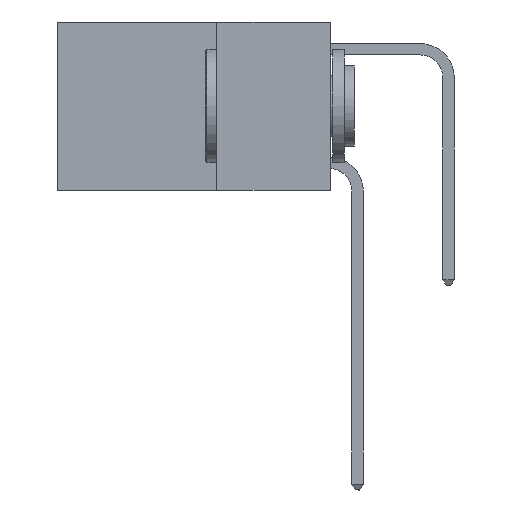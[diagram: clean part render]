
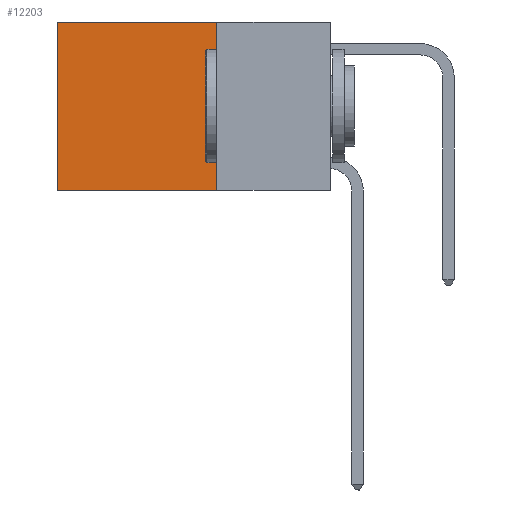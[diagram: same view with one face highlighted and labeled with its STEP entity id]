
A CAD part, left-side view. The second image highlights one B-rep face of the part: STEP entity #12203.
In plain terms, the highlighted planar face has unit normal (-1, 0, 0).
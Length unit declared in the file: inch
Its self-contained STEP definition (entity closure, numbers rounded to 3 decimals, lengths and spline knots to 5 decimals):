
#257 = AXIS2_PLACEMENT_3D ( 'NONE', #25363, #6203, #25507 ) ;
#851 = EDGE_CURVE ( 'NONE', #8755, #5757, #17327, .T. ) ;
#964 = VERTEX_POINT ( 'NONE', #20025 ) ;
#1953 = ORIENTED_EDGE ( 'NONE', *, *, #21762, .T. ) ;
#2102 = EDGE_LOOP ( 'NONE', ( #1953, #13893, #17012, #3191 ) ) ;
#3191 = ORIENTED_EDGE ( 'NONE', *, *, #851, .T. ) ;
#4063 = PLANE ( 'NONE',  #257 ) ;
#4317 = DIRECTION ( 'NONE',  ( 0., 1., 0. ) ) ;
#5757 = VERTEX_POINT ( 'NONE', #9289 ) ;
#6203 = DIRECTION ( 'NONE',  ( 1., 0., 0. ) ) ;
#8755 = VERTEX_POINT ( 'NONE', #10433 ) ;
#9289 = CARTESIAN_POINT ( 'NONE',  ( 0.2625, 0.6, 0. ) ) ;
#9304 = CARTESIAN_POINT ( 'NONE',  ( 0.2625, 0.6, 0. ) ) ;
#10433 = CARTESIAN_POINT ( 'NONE',  ( 0.2625, 0.25, 0. ) ) ;
#11024 = DIRECTION ( 'NONE',  ( 0., 0., -1. ) ) ;
#12203 = ADVANCED_FACE ( 'NONE', ( #19207 ), #4063, .F. ) ;
#12330 = LINE ( 'NONE', #16619, #22989 ) ;
#13893 = ORIENTED_EDGE ( 'NONE', *, *, #19426, .F. ) ;
#15647 = LINE ( 'NONE', #16073, #24967 ) ;
#16073 = CARTESIAN_POINT ( 'NONE',  ( 0.2625, 0.25, -0.37 ) ) ;
#16619 = CARTESIAN_POINT ( 'NONE',  ( 0.2625, 0.25, 0. ) ) ;
#17012 = ORIENTED_EDGE ( 'NONE', *, *, #26315, .F. ) ;
#17327 = LINE ( 'NONE', #26048, #18601 ) ;
#17755 = CARTESIAN_POINT ( 'NONE',  ( 0.2625, 0.25, -0.37 ) ) ;
#18601 = VECTOR ( 'NONE', #4317, 39.37008 ) ;
#18914 = DIRECTION ( 'NONE',  ( 0., 0., -1. ) ) ;
#19207 = FACE_OUTER_BOUND ( 'NONE', #2102, .T. ) ;
#19232 = VECTOR ( 'NONE', #11024, 39.37008 ) ;
#19426 = EDGE_CURVE ( 'NONE', #25204, #964, #15647, .T. ) ;
#20025 = CARTESIAN_POINT ( 'NONE',  ( 0.2625, 0.6, -0.37 ) ) ;
#21762 = EDGE_CURVE ( 'NONE', #5757, #964, #24042, .T. ) ;
#22511 = DIRECTION ( 'NONE',  ( 0., 1., 0. ) ) ;
#22989 = VECTOR ( 'NONE', #18914, 39.37008 ) ;
#24042 = LINE ( 'NONE', #9304, #19232 ) ;
#24967 = VECTOR ( 'NONE', #22511, 39.37008 ) ;
#25204 = VERTEX_POINT ( 'NONE', #17755 ) ;
#25363 = CARTESIAN_POINT ( 'NONE',  ( 0.2625, 0.25, 0. ) ) ;
#25507 = DIRECTION ( 'NONE',  ( 0., 0., -1. ) ) ;
#26048 = CARTESIAN_POINT ( 'NONE',  ( 0.2625, 0.25, 0. ) ) ;
#26315 = EDGE_CURVE ( 'NONE', #8755, #25204, #12330, .T. ) ;
